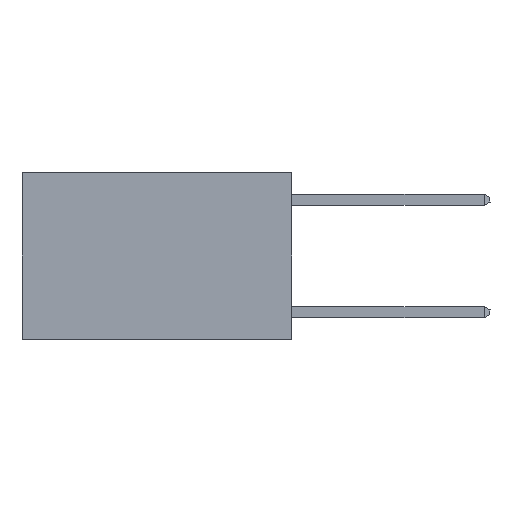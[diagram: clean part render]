
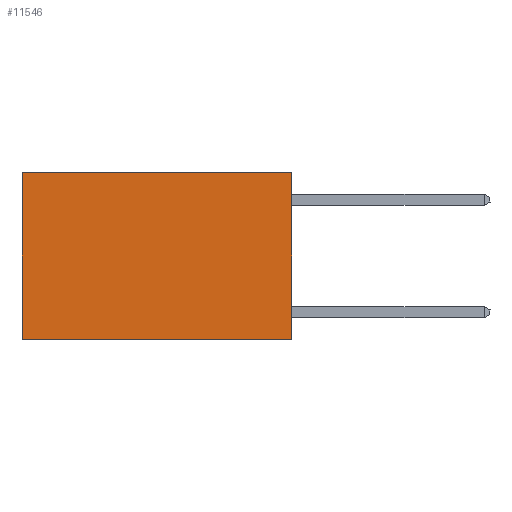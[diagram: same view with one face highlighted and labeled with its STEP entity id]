
A CAD part, left-side view. The second image highlights one B-rep face of the part: STEP entity #11546.
In plain terms, the highlighted planar face has unit normal (-1, 0, 0).
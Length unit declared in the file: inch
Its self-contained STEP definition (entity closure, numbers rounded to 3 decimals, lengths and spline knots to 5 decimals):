
#182 = CARTESIAN_POINT ( 'NONE',  ( 0.2625, 0.6, 0. ) ) ;
#732 = EDGE_LOOP ( 'NONE', ( #12567, #14320, #4642, #19413 ) ) ;
#1147 = VECTOR ( 'NONE', #10913, 39.37008 ) ;
#3930 = DIRECTION ( 'NONE',  ( 0., 0., -1. ) ) ;
#4642 = ORIENTED_EDGE ( 'NONE', *, *, #6307, .F. ) ;
#5189 = LINE ( 'NONE', #20291, #6913 ) ;
#6307 = EDGE_CURVE ( 'NONE', #14383, #13760, #14831, .T. ) ;
#6423 = DIRECTION ( 'NONE',  ( 0., 0., -1. ) ) ;
#6793 = VERTEX_POINT ( 'NONE', #12712 ) ;
#6842 = DIRECTION ( 'NONE',  ( 1., 0., 0. ) ) ;
#6913 = VECTOR ( 'NONE', #7753, 39.37008 ) ;
#6968 = PLANE ( 'NONE',  #12091 ) ;
#7753 = DIRECTION ( 'NONE',  ( 0., 1., 0. ) ) ;
#9742 = CARTESIAN_POINT ( 'NONE',  ( 0.2625, 0., -0.37 ) ) ;
#10489 = LINE ( 'NONE', #12300, #1147 ) ;
#10913 = DIRECTION ( 'NONE',  ( 0., 1., 0. ) ) ;
#11546 = ADVANCED_FACE ( 'NONE', ( #12213 ), #6968, .F. ) ;
#12091 = AXIS2_PLACEMENT_3D ( 'NONE', #14715, #6842, #16517 ) ;
#12135 = LINE ( 'NONE', #182, #14860 ) ;
#12213 = FACE_OUTER_BOUND ( 'NONE', #732, .T. ) ;
#12268 = EDGE_CURVE ( 'NONE', #13760, #18450, #10489, .T. ) ;
#12300 = CARTESIAN_POINT ( 'NONE',  ( 0.2625, 0., -0.37 ) ) ;
#12567 = ORIENTED_EDGE ( 'NONE', *, *, #13724, .T. ) ;
#12712 = CARTESIAN_POINT ( 'NONE',  ( 0.2625, 0.6, 0. ) ) ;
#12827 = VECTOR ( 'NONE', #3930, 39.37008 ) ;
#13138 = CARTESIAN_POINT ( 'NONE',  ( 0.2625, 0., 0. ) ) ;
#13724 = EDGE_CURVE ( 'NONE', #6793, #18450, #12135, .T. ) ;
#13760 = VERTEX_POINT ( 'NONE', #9742 ) ;
#14280 = CARTESIAN_POINT ( 'NONE',  ( 0.2625, 0., 0. ) ) ;
#14320 = ORIENTED_EDGE ( 'NONE', *, *, #12268, .F. ) ;
#14383 = VERTEX_POINT ( 'NONE', #14280 ) ;
#14715 = CARTESIAN_POINT ( 'NONE',  ( 0.2625, 0., 0. ) ) ;
#14831 = LINE ( 'NONE', #13138, #12827 ) ;
#14860 = VECTOR ( 'NONE', #6423, 39.37008 ) ;
#15052 = CARTESIAN_POINT ( 'NONE',  ( 0.2625, 0.6, -0.37 ) ) ;
#15053 = EDGE_CURVE ( 'NONE', #14383, #6793, #5189, .T. ) ;
#16517 = DIRECTION ( 'NONE',  ( 0., 0., -1. ) ) ;
#18450 = VERTEX_POINT ( 'NONE', #15052 ) ;
#19413 = ORIENTED_EDGE ( 'NONE', *, *, #15053, .T. ) ;
#20291 = CARTESIAN_POINT ( 'NONE',  ( 0.2625, 0., 0. ) ) ;
